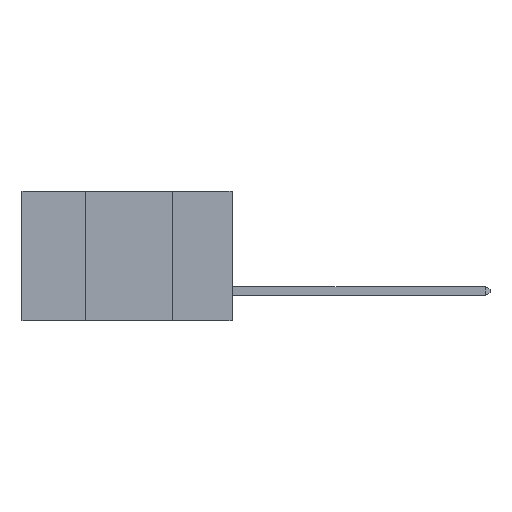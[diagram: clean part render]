
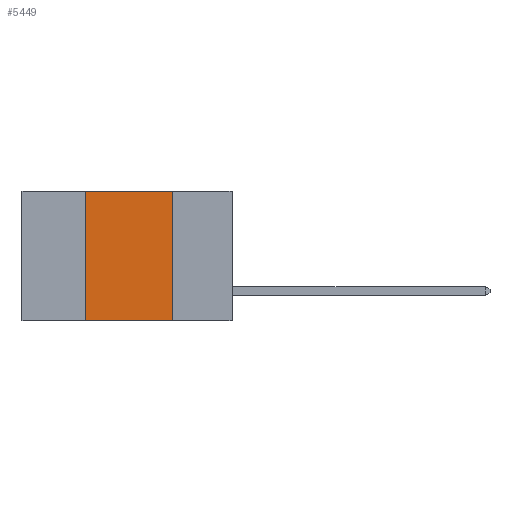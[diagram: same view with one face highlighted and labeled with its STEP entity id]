
A CAD part, left-side view. The second image highlights one B-rep face of the part: STEP entity #5449.
In plain terms, the highlighted planar face has unit normal (-1, 0, 0).
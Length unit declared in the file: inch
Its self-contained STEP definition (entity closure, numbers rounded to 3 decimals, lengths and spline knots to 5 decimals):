
#197 = DIRECTION ( 'NONE',  ( 0., 0., -1. ) ) ;
#299 = ORIENTED_EDGE ( 'NONE', *, *, #759, .T. ) ;
#759 = EDGE_CURVE ( 'NONE', #21001, #12175, #10679, .T. ) ;
#1492 = LINE ( 'NONE', #9885, #16247 ) ;
#2171 = VECTOR ( 'NONE', #24497, 39.37008 ) ;
#3095 = FACE_OUTER_BOUND ( 'NONE', #17601, .T. ) ;
#3311 = DIRECTION ( 'NONE',  ( 0., -1., 0. ) ) ;
#3602 = CARTESIAN_POINT ( 'NONE',  ( 0., 0.42, 0. ) ) ;
#5185 = VECTOR ( 'NONE', #3311, 39.37008 ) ;
#5293 = CARTESIAN_POINT ( 'NONE',  ( 0., 0.17, 0. ) ) ;
#5449 = ADVANCED_FACE ( 'NONE', ( #3095 ), #12847, .F. ) ;
#7788 = LINE ( 'NONE', #20310, #2171 ) ;
#7835 = DIRECTION ( 'NONE',  ( 0., 0., 1. ) ) ;
#8196 = CARTESIAN_POINT ( 'NONE',  ( 0., 0.6, 0. ) ) ;
#8694 = VERTEX_POINT ( 'NONE', #3602 ) ;
#8959 = ORIENTED_EDGE ( 'NONE', *, *, #12924, .F. ) ;
#9885 = CARTESIAN_POINT ( 'NONE',  ( 0., 0.42, 0. ) ) ;
#10407 = CARTESIAN_POINT ( 'NONE',  ( 0., 0.42, -0.37 ) ) ;
#10679 = LINE ( 'NONE', #17745, #5185 ) ;
#10768 = CARTESIAN_POINT ( 'NONE',  ( 0., 0.6, 0. ) ) ;
#12175 = VERTEX_POINT ( 'NONE', #21361 ) ;
#12847 = PLANE ( 'NONE',  #20951 ) ;
#12924 = EDGE_CURVE ( 'NONE', #17516, #12175, #7788, .T. ) ;
#15669 = LINE ( 'NONE', #8196, #20585 ) ;
#15783 = EDGE_CURVE ( 'NONE', #8694, #17516, #15669, .T. ) ;
#16247 = VECTOR ( 'NONE', #7835, 39.37008 ) ;
#16471 = ORIENTED_EDGE ( 'NONE', *, *, #17675, .F. ) ;
#17516 = VERTEX_POINT ( 'NONE', #5293 ) ;
#17601 = EDGE_LOOP ( 'NONE', ( #8959, #20744, #16471, #299 ) ) ;
#17675 = EDGE_CURVE ( 'NONE', #21001, #8694, #1492, .T. ) ;
#17745 = CARTESIAN_POINT ( 'NONE',  ( 0., 0.6, -0.37 ) ) ;
#18581 = DIRECTION ( 'NONE',  ( 0., -1., 0. ) ) ;
#19088 = DIRECTION ( 'NONE',  ( 1., 0., 0. ) ) ;
#20310 = CARTESIAN_POINT ( 'NONE',  ( 0., 0.17, 0. ) ) ;
#20585 = VECTOR ( 'NONE', #18581, 39.37008 ) ;
#20744 = ORIENTED_EDGE ( 'NONE', *, *, #15783, .F. ) ;
#20951 = AXIS2_PLACEMENT_3D ( 'NONE', #10768, #19088, #197 ) ;
#21001 = VERTEX_POINT ( 'NONE', #10407 ) ;
#21361 = CARTESIAN_POINT ( 'NONE',  ( 0., 0.17, -0.37 ) ) ;
#24497 = DIRECTION ( 'NONE',  ( 0., 0., -1. ) ) ;
